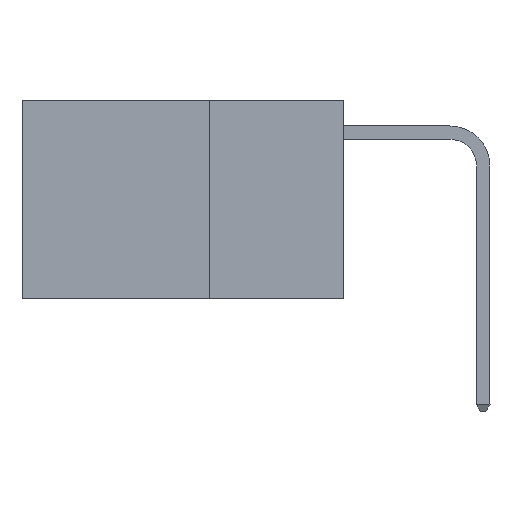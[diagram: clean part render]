
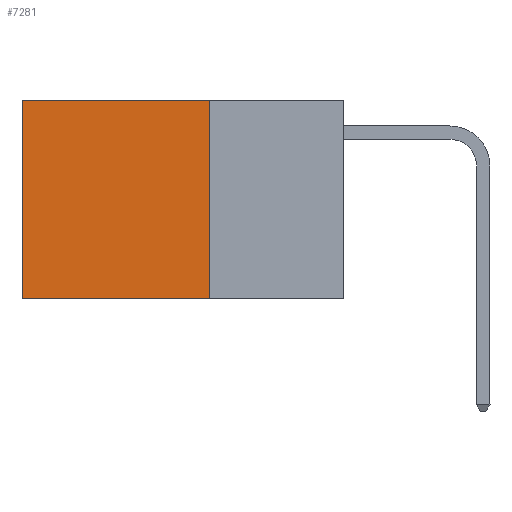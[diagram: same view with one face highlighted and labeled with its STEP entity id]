
A CAD part, left-side view. The second image highlights one B-rep face of the part: STEP entity #7281.
In plain terms, the highlighted planar face has unit normal (-1, 0, 0).
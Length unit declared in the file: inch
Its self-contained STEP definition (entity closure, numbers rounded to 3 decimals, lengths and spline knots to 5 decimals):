
#306 = AXIS2_PLACEMENT_3D ( 'NONE', #10544, #315, #7195 ) ;
#315 = DIRECTION ( 'NONE',  ( 1., 0., 0. ) ) ;
#942 = EDGE_CURVE ( 'NONE', #4963, #5263, #3755, .T. ) ;
#2130 = FACE_OUTER_BOUND ( 'NONE', #6150, .T. ) ;
#2238 = DIRECTION ( 'NONE',  ( 0., 0., -1. ) ) ;
#2341 = VECTOR ( 'NONE', #8335, 39.37008 ) ;
#2515 = VECTOR ( 'NONE', #9137, 39.37008 ) ;
#3049 = DIRECTION ( 'NONE',  ( 0., 1., 0. ) ) ;
#3515 = LINE ( 'NONE', #8636, #11024 ) ;
#3755 = LINE ( 'NONE', #7916, #7068 ) ;
#4004 = EDGE_CURVE ( 'NONE', #5263, #8302, #6361, .T. ) ;
#4323 = ORIENTED_EDGE ( 'NONE', *, *, #6750, .F. ) ;
#4592 = EDGE_CURVE ( 'NONE', #6487, #8302, #4646, .T. ) ;
#4646 = LINE ( 'NONE', #8197, #2341 ) ;
#4963 = VERTEX_POINT ( 'NONE', #9880 ) ;
#5263 = VERTEX_POINT ( 'NONE', #6868 ) ;
#5613 = ORIENTED_EDGE ( 'NONE', *, *, #4004, .T. ) ;
#6150 = EDGE_LOOP ( 'NONE', ( #5613, #10898, #4323, #7138 ) ) ;
#6361 = LINE ( 'NONE', #7745, #2515 ) ;
#6487 = VERTEX_POINT ( 'NONE', #10177 ) ;
#6750 = EDGE_CURVE ( 'NONE', #4963, #6487, #3515, .T. ) ;
#6868 = CARTESIAN_POINT ( 'NONE',  ( 0.2625, 0.6, 0. ) ) ;
#7068 = VECTOR ( 'NONE', #3049, 39.37008 ) ;
#7138 = ORIENTED_EDGE ( 'NONE', *, *, #942, .T. ) ;
#7195 = DIRECTION ( 'NONE',  ( 0., 0., -1. ) ) ;
#7281 = ADVANCED_FACE ( 'NONE', ( #2130 ), #8453, .F. ) ;
#7745 = CARTESIAN_POINT ( 'NONE',  ( 0.2625, 0.6, 0. ) ) ;
#7916 = CARTESIAN_POINT ( 'NONE',  ( 0.2625, 0.25, 0. ) ) ;
#8197 = CARTESIAN_POINT ( 'NONE',  ( 0.2625, 0.25, -0.37 ) ) ;
#8302 = VERTEX_POINT ( 'NONE', #8861 ) ;
#8335 = DIRECTION ( 'NONE',  ( 0., 1., 0. ) ) ;
#8453 = PLANE ( 'NONE',  #306 ) ;
#8636 = CARTESIAN_POINT ( 'NONE',  ( 0.2625, 0.25, 0. ) ) ;
#8861 = CARTESIAN_POINT ( 'NONE',  ( 0.2625, 0.6, -0.37 ) ) ;
#9137 = DIRECTION ( 'NONE',  ( 0., 0., -1. ) ) ;
#9880 = CARTESIAN_POINT ( 'NONE',  ( 0.2625, 0.25, 0. ) ) ;
#10177 = CARTESIAN_POINT ( 'NONE',  ( 0.2625, 0.25, -0.37 ) ) ;
#10544 = CARTESIAN_POINT ( 'NONE',  ( 0.2625, 0.25, 0. ) ) ;
#10898 = ORIENTED_EDGE ( 'NONE', *, *, #4592, .F. ) ;
#11024 = VECTOR ( 'NONE', #2238, 39.37008 ) ;
